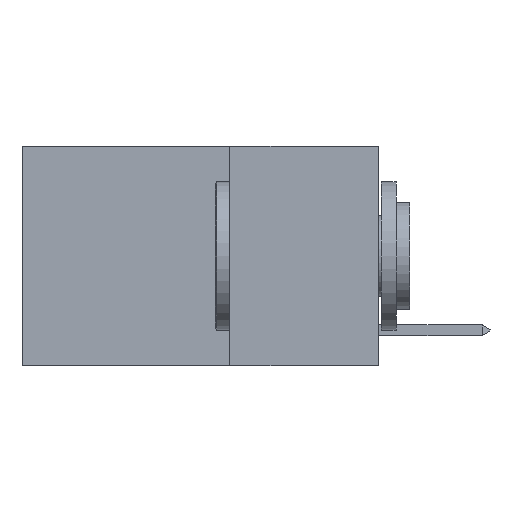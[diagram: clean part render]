
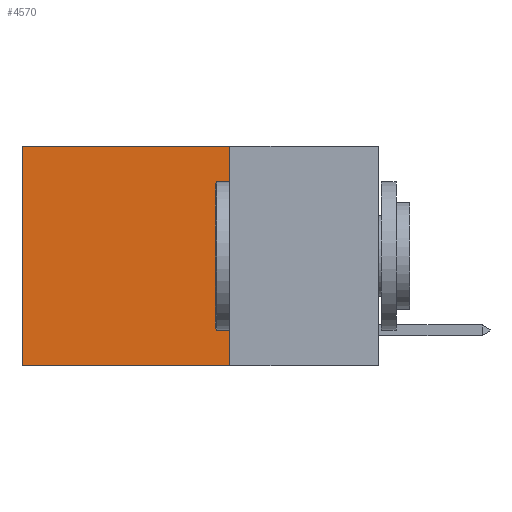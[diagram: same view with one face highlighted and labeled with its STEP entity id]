
A CAD part, left-side view. The second image highlights one B-rep face of the part: STEP entity #4570.
In plain terms, the highlighted planar face has unit normal (-1, 0, 0).
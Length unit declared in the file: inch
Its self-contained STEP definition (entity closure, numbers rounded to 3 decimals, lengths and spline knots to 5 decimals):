
#274 = ORIENTED_EDGE ( 'NONE', *, *, #11076, .T. ) ;
#676 = FACE_OUTER_BOUND ( 'NONE', #8140, .T. ) ;
#1112 = DIRECTION ( 'NONE',  ( 0., 0., -1. ) ) ;
#1958 = EDGE_CURVE ( 'NONE', #18881, #3661, #13140, .T. ) ;
#2361 = PLANE ( 'NONE',  #3386 ) ;
#2573 = CARTESIAN_POINT ( 'NONE',  ( 0.2625, 0.25, 0. ) ) ;
#2707 = LINE ( 'NONE', #8581, #13435 ) ;
#3386 = AXIS2_PLACEMENT_3D ( 'NONE', #18626, #5411, #6714 ) ;
#3661 = VERTEX_POINT ( 'NONE', #11560 ) ;
#4253 = DIRECTION ( 'NONE',  ( 0., 1., 0. ) ) ;
#4433 = DIRECTION ( 'NONE',  ( 0., 0., -1. ) ) ;
#4570 = ADVANCED_FACE ( 'NONE', ( #676 ), #2361, .F. ) ;
#5021 = ORIENTED_EDGE ( 'NONE', *, *, #15310, .F. ) ;
#5197 = ORIENTED_EDGE ( 'NONE', *, *, #1958, .F. ) ;
#5411 = DIRECTION ( 'NONE',  ( 1., 0., 0. ) ) ;
#6714 = DIRECTION ( 'NONE',  ( 0., 0., -1. ) ) ;
#6851 = CARTESIAN_POINT ( 'NONE',  ( 0.2625, 0.6, 0. ) ) ;
#7044 = CARTESIAN_POINT ( 'NONE',  ( 0.2625, 0.25, 0. ) ) ;
#7076 = DIRECTION ( 'NONE',  ( 0., 1., 0. ) ) ;
#7271 = EDGE_CURVE ( 'NONE', #15943, #9018, #11685, .T. ) ;
#8140 = EDGE_LOOP ( 'NONE', ( #8718, #5021, #5197, #274 ) ) ;
#8581 = CARTESIAN_POINT ( 'NONE',  ( 0.2625, 0.25, -0.37 ) ) ;
#8718 = ORIENTED_EDGE ( 'NONE', *, *, #7271, .T. ) ;
#9018 = VERTEX_POINT ( 'NONE', #12554 ) ;
#11076 = EDGE_CURVE ( 'NONE', #18881, #15943, #18922, .T. ) ;
#11560 = CARTESIAN_POINT ( 'NONE',  ( 0.2625, 0.25, -0.37 ) ) ;
#11685 = LINE ( 'NONE', #6851, #16090 ) ;
#12134 = CARTESIAN_POINT ( 'NONE',  ( 0.2625, 0.6, 0. ) ) ;
#12554 = CARTESIAN_POINT ( 'NONE',  ( 0.2625, 0.6, -0.37 ) ) ;
#12654 = VECTOR ( 'NONE', #4253, 39.37008 ) ;
#13140 = LINE ( 'NONE', #2573, #15675 ) ;
#13435 = VECTOR ( 'NONE', #7076, 39.37008 ) ;
#15310 = EDGE_CURVE ( 'NONE', #3661, #9018, #2707, .T. ) ;
#15675 = VECTOR ( 'NONE', #4433, 39.37008 ) ;
#15943 = VERTEX_POINT ( 'NONE', #12134 ) ;
#16090 = VECTOR ( 'NONE', #1112, 39.37008 ) ;
#17763 = CARTESIAN_POINT ( 'NONE',  ( 0.2625, 0.25, 0. ) ) ;
#18626 = CARTESIAN_POINT ( 'NONE',  ( 0.2625, 0.25, 0. ) ) ;
#18881 = VERTEX_POINT ( 'NONE', #7044 ) ;
#18922 = LINE ( 'NONE', #17763, #12654 ) ;
